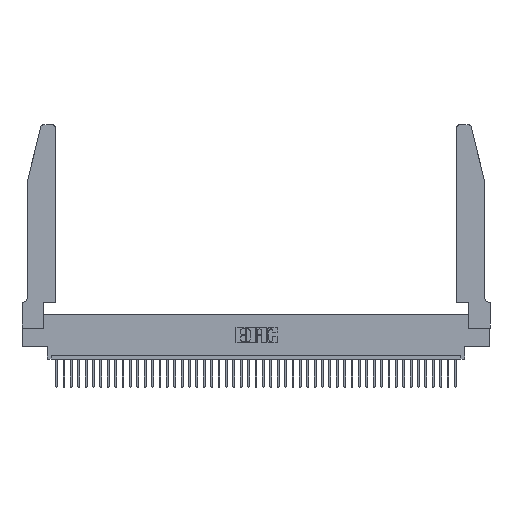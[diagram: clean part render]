
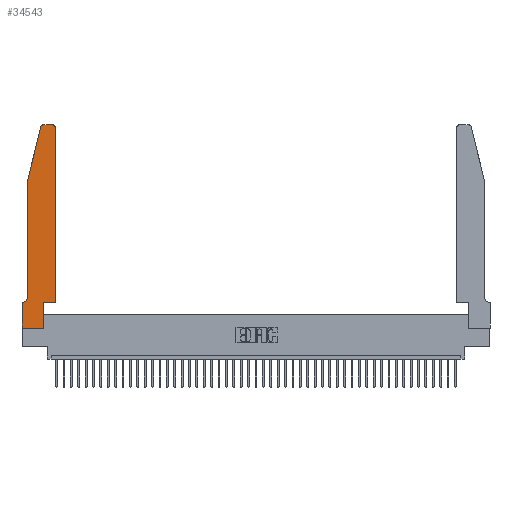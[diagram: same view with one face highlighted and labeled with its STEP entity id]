
A CAD part, top view. The second image highlights one B-rep face of the part: STEP entity #34543.
In plain terms, the highlighted planar face has unit normal (0, 0, 1).
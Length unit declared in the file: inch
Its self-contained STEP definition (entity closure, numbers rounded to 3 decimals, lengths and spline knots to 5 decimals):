
#1110 = CARTESIAN_POINT ( 'NONE',  ( 0.4505, 0.35, 0.37 ) ) ;
#1287 = CARTESIAN_POINT ( 'NONE',  ( 0.0755, 0.42, 0.37 ) ) ;
#1332 = DIRECTION ( 'NONE',  ( 1., 0., 0. ) ) ;
#2088 = CARTESIAN_POINT ( 'NONE',  ( 0., 0., 0.37 ) ) ;
#2130 = VECTOR ( 'NONE', #5723, 39.37008 ) ;
#2179 = CARTESIAN_POINT ( 'NONE',  ( 0.0755, 2., 0.37 ) ) ;
#4470 = CARTESIAN_POINT ( 'NONE',  ( 0.0755, 0.35, 0.37 ) ) ;
#4809 = DIRECTION ( 'NONE',  ( 0., 0., 1. ) ) ;
#5174 = CARTESIAN_POINT ( 'NONE',  ( 0., 0., 0.37 ) ) ;
#5723 = DIRECTION ( 'NONE',  ( 1., 0., 0. ) ) ;
#7474 = ORIENTED_EDGE ( 'NONE', *, *, #15787, .T. ) ;
#7574 = ORIENTED_EDGE ( 'NONE', *, *, #13747, .T. ) ;
#7806 = DIRECTION ( 'NONE',  ( 0., 0., 1. ) ) ;
#8327 = CARTESIAN_POINT ( 'NONE',  ( 0.2865, 0., 0.37 ) ) ;
#8716 = ORIENTED_EDGE ( 'NONE', *, *, #16754, .T. ) ;
#8889 = CARTESIAN_POINT ( 'NONE',  ( 0.0755, 2., 0.37 ) ) ;
#9184 = CARTESIAN_POINT ( 'NONE',  ( 0.25487, 2.72718, 0.37 ) ) ;
#9494 = CARTESIAN_POINT ( 'NONE',  ( 0.4505, 0.35, 0.37 ) ) ;
#9783 = EDGE_CURVE ( 'NONE', #19270, #11403, #17392, .T. ) ;
#9790 = VERTEX_POINT ( 'NONE', #25391 ) ;
#10265 = EDGE_CURVE ( 'NONE', #27253, #19270, #29172, .T. ) ;
#10740 = CARTESIAN_POINT ( 'NONE',  ( 0.4205, 2.75, 0.37 ) ) ;
#11089 = VECTOR ( 'NONE', #42199, 39.37008 ) ;
#11403 = VERTEX_POINT ( 'NONE', #10740 ) ;
#12054 = CIRCLE ( 'NONE', #32488, 0.03 ) ;
#12575 = AXIS2_PLACEMENT_3D ( 'NONE', #21801, #42819, #21953 ) ;
#12975 = ORIENTED_EDGE ( 'NONE', *, *, #43426, .T. ) ;
#13747 = EDGE_CURVE ( 'NONE', #32213, #27253, #34404, .T. ) ;
#14403 = DIRECTION ( 'NONE',  ( 1., 0., 0. ) ) ;
#15787 = EDGE_CURVE ( 'NONE', #36241, #18578, #24540, .T. ) ;
#16754 = EDGE_CURVE ( 'NONE', #9790, #32746, #12054, .T. ) ;
#16908 = ORIENTED_EDGE ( 'NONE', *, *, #10265, .T. ) ;
#16940 = CARTESIAN_POINT ( 'NONE',  ( 0., 0.35, 0.37 ) ) ;
#17392 = CIRCLE ( 'NONE', #43533, 0.03 ) ;
#17901 = CARTESIAN_POINT ( 'NONE',  ( 0.4505, 2.72, 0.37 ) ) ;
#18176 = FACE_OUTER_BOUND ( 'NONE', #26148, .T. ) ;
#18480 = CARTESIAN_POINT ( 'NONE',  ( 0.4205, 2.72, 0.37 ) ) ;
#18578 = VERTEX_POINT ( 'NONE', #21355 ) ;
#19028 = DIRECTION ( 'NONE',  ( -0.239, -0.971, 0. ) ) ;
#19257 = CARTESIAN_POINT ( 'NONE',  ( 0.2865, 0.35, 0.37 ) ) ;
#19270 = VERTEX_POINT ( 'NONE', #17901 ) ;
#19414 = CARTESIAN_POINT ( 'NONE',  ( 0., 0., 0.37 ) ) ;
#20307 = LINE ( 'NONE', #22296, #22516 ) ;
#20746 = VECTOR ( 'NONE', #32937, 39.37008 ) ;
#21090 = VECTOR ( 'NONE', #37838, 39.37008 ) ;
#21163 = CARTESIAN_POINT ( 'NONE',  ( 0.284, 2.72, 0.37 ) ) ;
#21355 = CARTESIAN_POINT ( 'NONE',  ( 0.0055, 0.35, 0.37 ) ) ;
#21365 = ORIENTED_EDGE ( 'NONE', *, *, #9783, .T. ) ;
#21801 = CARTESIAN_POINT ( 'NONE',  ( 0.0055, 0.42, 0.37 ) ) ;
#21953 = DIRECTION ( 'NONE',  ( -1., 0., 0. ) ) ;
#21973 = ORIENTED_EDGE ( 'NONE', *, *, #44069, .T. ) ;
#22296 = CARTESIAN_POINT ( 'NONE',  ( 0.2865, 0.35, 0.37 ) ) ;
#22436 = ORIENTED_EDGE ( 'NONE', *, *, #34592, .T. ) ;
#22516 = VECTOR ( 'NONE', #39240, 39.37008 ) ;
#22577 = DIRECTION ( 'NONE',  ( 0., -1., 0. ) ) ;
#23159 = EDGE_CURVE ( 'NONE', #18578, #35890, #38469, .T. ) ;
#24540 = CIRCLE ( 'NONE', #12575, 0.07 ) ;
#24923 = DIRECTION ( 'NONE',  ( -1., 0., 0. ) ) ;
#25196 = VECTOR ( 'NONE', #24923, 39.37008 ) ;
#25391 = CARTESIAN_POINT ( 'NONE',  ( 0.284, 2.75, 0.37 ) ) ;
#25864 = CARTESIAN_POINT ( 'NONE',  ( 0.0755, 2., 0.37 ) ) ;
#26148 = EDGE_LOOP ( 'NONE', ( #42838, #8716, #21973, #12975, #7474, #35222, #22436, #33177, #35389, #7574, #16908, #21365 ) ) ;
#26155 = PLANE ( 'NONE',  #41781 ) ;
#26601 = DIRECTION ( 'NONE',  ( 0., 0., 1. ) ) ;
#26610 = CARTESIAN_POINT ( 'NONE',  ( 0.4505, 0.35, 0.37 ) ) ;
#26938 = LINE ( 'NONE', #2179, #39301 ) ;
#27253 = VERTEX_POINT ( 'NONE', #1110 ) ;
#29172 = LINE ( 'NONE', #9494, #21090 ) ;
#29480 = LINE ( 'NONE', #2088, #39661 ) ;
#31104 = EDGE_CURVE ( 'NONE', #32119, #32213, #20307, .T. ) ;
#32119 = VERTEX_POINT ( 'NONE', #8327 ) ;
#32213 = VERTEX_POINT ( 'NONE', #19257 ) ;
#32215 = LINE ( 'NONE', #38893, #25196 ) ;
#32488 = AXIS2_PLACEMENT_3D ( 'NONE', #21163, #7806, #14403 ) ;
#32746 = VERTEX_POINT ( 'NONE', #9184 ) ;
#32937 = DIRECTION ( 'NONE',  ( 0., -1., 0. ) ) ;
#33177 = ORIENTED_EDGE ( 'NONE', *, *, #40504, .T. ) ;
#33509 = CARTESIAN_POINT ( 'NONE',  ( 0., 0.35, 0.37 ) ) ;
#34404 = LINE ( 'NONE', #26610, #2130 ) ;
#34479 = VERTEX_POINT ( 'NONE', #25864 ) ;
#34543 = ADVANCED_FACE ( 'NONE', ( #18176 ), #26155, .T. ) ;
#34592 = EDGE_CURVE ( 'NONE', #35890, #44402, #29480, .T. ) ;
#34880 = EDGE_CURVE ( 'NONE', #11403, #9790, #32215, .T. ) ;
#35222 = ORIENTED_EDGE ( 'NONE', *, *, #23159, .T. ) ;
#35389 = ORIENTED_EDGE ( 'NONE', *, *, #31104, .T. ) ;
#35890 = VERTEX_POINT ( 'NONE', #16940 ) ;
#36241 = VERTEX_POINT ( 'NONE', #1287 ) ;
#37838 = DIRECTION ( 'NONE',  ( 0., 1., 0. ) ) ;
#38196 = LINE ( 'NONE', #19414, #44119 ) ;
#38469 = LINE ( 'NONE', #4470, #11089 ) ;
#38893 = CARTESIAN_POINT ( 'NONE',  ( 0.2605, 2.75, 0.37 ) ) ;
#39240 = DIRECTION ( 'NONE',  ( 0., 1., 0. ) ) ;
#39301 = VECTOR ( 'NONE', #19028, 39.37008 ) ;
#39661 = VECTOR ( 'NONE', #22577, 39.37008 ) ;
#40504 = EDGE_CURVE ( 'NONE', #44402, #32119, #38196, .T. ) ;
#40673 = LINE ( 'NONE', #8889, #20746 ) ;
#41781 = AXIS2_PLACEMENT_3D ( 'NONE', #33509, #26601, #43709 ) ;
#42199 = DIRECTION ( 'NONE',  ( -1., 0., 0. ) ) ;
#42819 = DIRECTION ( 'NONE',  ( 0., 0., -1. ) ) ;
#42838 = ORIENTED_EDGE ( 'NONE', *, *, #34880, .T. ) ;
#43426 = EDGE_CURVE ( 'NONE', #34479, #36241, #40673, .T. ) ;
#43533 = AXIS2_PLACEMENT_3D ( 'NONE', #18480, #4809, #1332 ) ;
#43709 = DIRECTION ( 'NONE',  ( 1., 0., 0. ) ) ;
#43888 = DIRECTION ( 'NONE',  ( 1., 0., 0. ) ) ;
#44069 = EDGE_CURVE ( 'NONE', #32746, #34479, #26938, .T. ) ;
#44119 = VECTOR ( 'NONE', #43888, 39.37008 ) ;
#44402 = VERTEX_POINT ( 'NONE', #5174 ) ;
